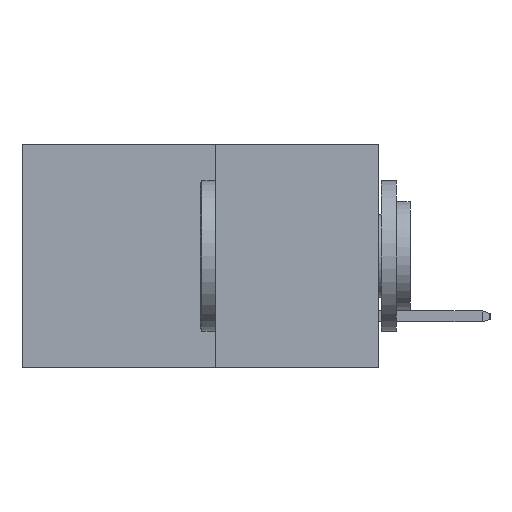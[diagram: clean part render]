
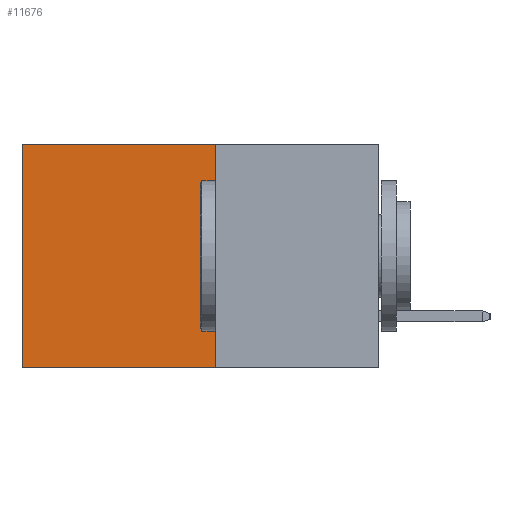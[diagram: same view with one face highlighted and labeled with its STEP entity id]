
A CAD part, left-side view. The second image highlights one B-rep face of the part: STEP entity #11676.
In plain terms, the highlighted planar face has unit normal (-1, 0, 0).
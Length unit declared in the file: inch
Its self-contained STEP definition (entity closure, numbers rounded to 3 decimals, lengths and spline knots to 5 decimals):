
#882 = VERTEX_POINT ( 'NONE', #10529 ) ;
#1232 = VERTEX_POINT ( 'NONE', #11483 ) ;
#1352 = DIRECTION ( 'NONE',  ( 0., 0., -1. ) ) ;
#1639 = LINE ( 'NONE', #8564, #6345 ) ;
#2151 = LINE ( 'NONE', #5229, #6811 ) ;
#2398 = ORIENTED_EDGE ( 'NONE', *, *, #4874, .T. ) ;
#2831 = ORIENTED_EDGE ( 'NONE', *, *, #8178, .F. ) ;
#3066 = ORIENTED_EDGE ( 'NONE', *, *, #11573, .T. ) ;
#3966 = CARTESIAN_POINT ( 'NONE',  ( 0.277, 0.59, -0.37 ) ) ;
#4044 = VERTEX_POINT ( 'NONE', #7327 ) ;
#4162 = EDGE_CURVE ( 'NONE', #1232, #4044, #2151, .T. ) ;
#4541 = CARTESIAN_POINT ( 'NONE',  ( 0.277, 0.59, 0. ) ) ;
#4551 = ORIENTED_EDGE ( 'NONE', *, *, #4162, .F. ) ;
#4581 = DIRECTION ( 'NONE',  ( 0., 0., -1. ) ) ;
#4674 = CARTESIAN_POINT ( 'NONE',  ( 0.277, 0.27, -0.37 ) ) ;
#4874 = EDGE_CURVE ( 'NONE', #7789, #4044, #6373, .T. ) ;
#4909 = FACE_OUTER_BOUND ( 'NONE', #11113, .T. ) ;
#5202 = DIRECTION ( 'NONE',  ( 0., 1., 0. ) ) ;
#5229 = CARTESIAN_POINT ( 'NONE',  ( 0.277, 0.27, -0.37 ) ) ;
#5230 = DIRECTION ( 'NONE',  ( 0., 0., -1. ) ) ;
#6061 = PLANE ( 'NONE',  #9508 ) ;
#6345 = VECTOR ( 'NONE', #9506, 39.37008 ) ;
#6373 = LINE ( 'NONE', #3966, #8760 ) ;
#6811 = VECTOR ( 'NONE', #5202, 39.37008 ) ;
#6951 = DIRECTION ( 'NONE',  ( 1., 0., 0. ) ) ;
#7327 = CARTESIAN_POINT ( 'NONE',  ( 0.277, 0.59, -0.37 ) ) ;
#7789 = VERTEX_POINT ( 'NONE', #4541 ) ;
#8115 = VECTOR ( 'NONE', #5230, 39.37008 ) ;
#8178 = EDGE_CURVE ( 'NONE', #882, #1232, #10536, .T. ) ;
#8564 = CARTESIAN_POINT ( 'NONE',  ( 0.277, 0.27, 0. ) ) ;
#8760 = VECTOR ( 'NONE', #4581, 39.37008 ) ;
#9506 = DIRECTION ( 'NONE',  ( 0., 1., 0. ) ) ;
#9508 = AXIS2_PLACEMENT_3D ( 'NONE', #11372, #6951, #1352 ) ;
#10529 = CARTESIAN_POINT ( 'NONE',  ( 0.277, 0.27, 0. ) ) ;
#10536 = LINE ( 'NONE', #4674, #8115 ) ;
#11113 = EDGE_LOOP ( 'NONE', ( #2398, #4551, #2831, #3066 ) ) ;
#11372 = CARTESIAN_POINT ( 'NONE',  ( 0.277, 0.27, -0.37 ) ) ;
#11483 = CARTESIAN_POINT ( 'NONE',  ( 0.277, 0.27, -0.37 ) ) ;
#11573 = EDGE_CURVE ( 'NONE', #882, #7789, #1639, .T. ) ;
#11676 = ADVANCED_FACE ( 'NONE', ( #4909 ), #6061, .F. ) ;
